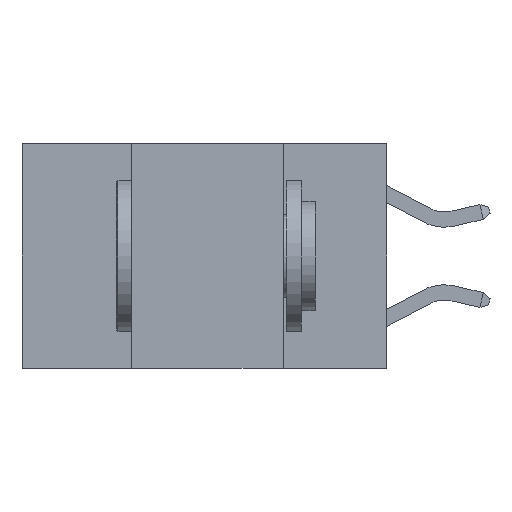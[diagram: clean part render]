
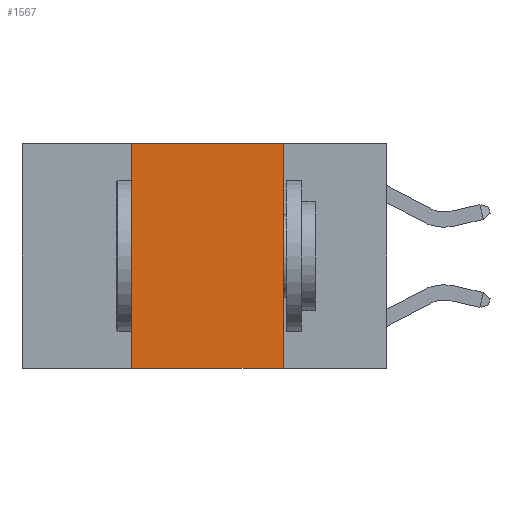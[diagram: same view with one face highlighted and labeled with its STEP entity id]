
A CAD part, left-side view. The second image highlights one B-rep face of the part: STEP entity #1567.
In plain terms, the highlighted planar face has unit normal (-1, 0, 0).
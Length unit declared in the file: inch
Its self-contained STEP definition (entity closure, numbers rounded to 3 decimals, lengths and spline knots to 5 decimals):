
#504 = EDGE_CURVE ( 'NONE', #14178, #5269, #14172, .T. ) ;
#942 = CARTESIAN_POINT ( 'NONE',  ( 0., 0.6, -0.37 ) ) ;
#1567 = ADVANCED_FACE ( 'NONE', ( #4931 ), #16818, .F. ) ;
#2369 = DIRECTION ( 'NONE',  ( 0., 0., -1. ) ) ;
#3714 = CARTESIAN_POINT ( 'NONE',  ( 0., 0.17, 0. ) ) ;
#4788 = EDGE_CURVE ( 'NONE', #14178, #14476, #15058, .T. ) ;
#4899 = LINE ( 'NONE', #3714, #5246 ) ;
#4931 = FACE_OUTER_BOUND ( 'NONE', #7504, .T. ) ;
#5021 = CARTESIAN_POINT ( 'NONE',  ( 0., 0.6, 0. ) ) ;
#5246 = VECTOR ( 'NONE', #2369, 39.37008 ) ;
#5269 = VERTEX_POINT ( 'NONE', #15762 ) ;
#6386 = EDGE_CURVE ( 'NONE', #14680, #5269, #4899, .T. ) ;
#7175 = AXIS2_PLACEMENT_3D ( 'NONE', #5021, #10251, #15535 ) ;
#7504 = EDGE_LOOP ( 'NONE', ( #8902, #16220, #14112, #8014 ) ) ;
#8014 = ORIENTED_EDGE ( 'NONE', *, *, #504, .T. ) ;
#8262 = CARTESIAN_POINT ( 'NONE',  ( 0., 0.42, 0. ) ) ;
#8902 = ORIENTED_EDGE ( 'NONE', *, *, #6386, .F. ) ;
#10251 = DIRECTION ( 'NONE',  ( 1., 0., 0. ) ) ;
#11290 = DIRECTION ( 'NONE',  ( 0., -1., 0. ) ) ;
#11428 = VECTOR ( 'NONE', #15552, 39.37008 ) ;
#11921 = CARTESIAN_POINT ( 'NONE',  ( 0., 0.42, -0.37 ) ) ;
#13755 = CARTESIAN_POINT ( 'NONE',  ( 0., 0.42, 0. ) ) ;
#14112 = ORIENTED_EDGE ( 'NONE', *, *, #4788, .F. ) ;
#14172 = LINE ( 'NONE', #942, #16886 ) ;
#14178 = VERTEX_POINT ( 'NONE', #11921 ) ;
#14429 = LINE ( 'NONE', #15702, #11428 ) ;
#14471 = CARTESIAN_POINT ( 'NONE',  ( 0., 0.17, 0. ) ) ;
#14476 = VERTEX_POINT ( 'NONE', #8262 ) ;
#14680 = VERTEX_POINT ( 'NONE', #14471 ) ;
#14948 = VECTOR ( 'NONE', #15143, 39.37008 ) ;
#15058 = LINE ( 'NONE', #13755, #14948 ) ;
#15143 = DIRECTION ( 'NONE',  ( 0., 0., 1. ) ) ;
#15535 = DIRECTION ( 'NONE',  ( 0., 0., -1. ) ) ;
#15552 = DIRECTION ( 'NONE',  ( 0., -1., 0. ) ) ;
#15702 = CARTESIAN_POINT ( 'NONE',  ( 0., 0.6, 0. ) ) ;
#15762 = CARTESIAN_POINT ( 'NONE',  ( 0., 0.17, -0.37 ) ) ;
#16072 = EDGE_CURVE ( 'NONE', #14476, #14680, #14429, .T. ) ;
#16220 = ORIENTED_EDGE ( 'NONE', *, *, #16072, .F. ) ;
#16818 = PLANE ( 'NONE',  #7175 ) ;
#16886 = VECTOR ( 'NONE', #11290, 39.37008 ) ;
